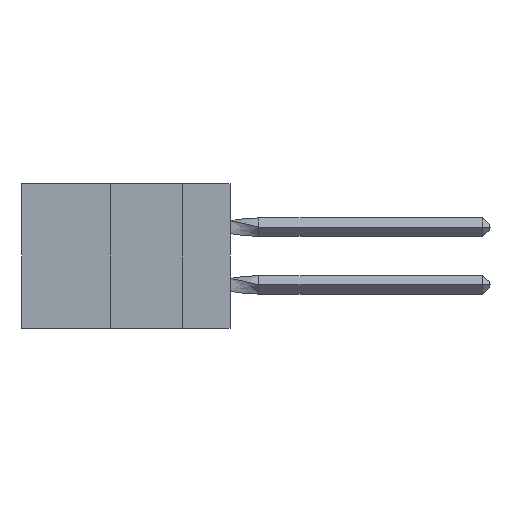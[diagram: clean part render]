
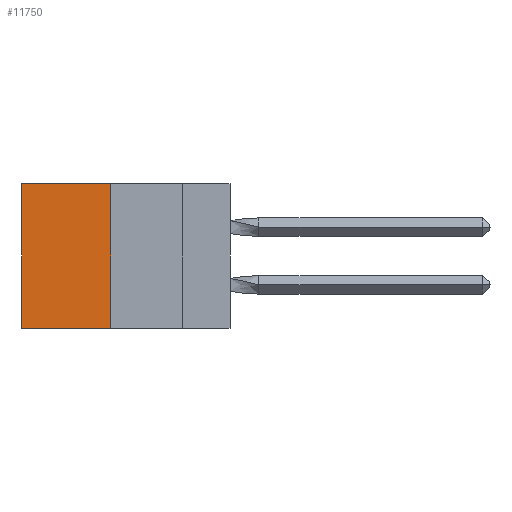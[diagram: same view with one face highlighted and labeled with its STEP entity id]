
A CAD part, left-side view. The second image highlights one B-rep face of the part: STEP entity #11750.
In plain terms, the highlighted planar face has unit normal (-1, 0, 0).
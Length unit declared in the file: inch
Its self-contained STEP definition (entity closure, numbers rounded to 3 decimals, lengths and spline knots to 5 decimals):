
#335 = DIRECTION ( 'NONE',  ( 0., 1., 0. ) ) ;
#405 = ORIENTED_EDGE ( 'NONE', *, *, #6622, .T. ) ;
#2825 = EDGE_CURVE ( 'NONE', #12807, #5251, #27028, .T. ) ;
#3251 = PLANE ( 'NONE',  #20923 ) ;
#3569 = DIRECTION ( 'NONE',  ( 0., 1., 0. ) ) ;
#4376 = CARTESIAN_POINT ( 'NONE',  ( 0.305, 0.413, -0.5 ) ) ;
#5109 = VERTEX_POINT ( 'NONE', #4376 ) ;
#5149 = CARTESIAN_POINT ( 'NONE',  ( 0.305, 0.72, 0. ) ) ;
#5251 = VERTEX_POINT ( 'NONE', #5149 ) ;
#6622 = EDGE_CURVE ( 'NONE', #5251, #14571, #18319, .T. ) ;
#6667 = VECTOR ( 'NONE', #20431, 39.37008 ) ;
#6891 = FACE_OUTER_BOUND ( 'NONE', #33500, .T. ) ;
#8095 = CARTESIAN_POINT ( 'NONE',  ( 0.305, 0.413, -0.5 ) ) ;
#10696 = EDGE_CURVE ( 'NONE', #5109, #14571, #30036, .T. ) ;
#11024 = CARTESIAN_POINT ( 'NONE',  ( 0.305, 0.413, -0.5 ) ) ;
#11435 = VECTOR ( 'NONE', #13709, 39.37008 ) ;
#11750 = ADVANCED_FACE ( 'NONE', ( #6891 ), #3251, .F. ) ;
#12391 = CARTESIAN_POINT ( 'NONE',  ( 0.305, 0.72, -0.5 ) ) ;
#12807 = VERTEX_POINT ( 'NONE', #29719 ) ;
#13709 = DIRECTION ( 'NONE',  ( 0., 0., -1. ) ) ;
#14567 = ORIENTED_EDGE ( 'NONE', *, *, #19750, .F. ) ;
#14571 = VERTEX_POINT ( 'NONE', #28990 ) ;
#17619 = LINE ( 'NONE', #11024, #11435 ) ;
#18319 = LINE ( 'NONE', #12391, #6667 ) ;
#19567 = VECTOR ( 'NONE', #335, 39.37008 ) ;
#19750 = EDGE_CURVE ( 'NONE', #12807, #5109, #17619, .T. ) ;
#20431 = DIRECTION ( 'NONE',  ( 0., 0., -1. ) ) ;
#20923 = AXIS2_PLACEMENT_3D ( 'NONE', #29618, #32327, #29840 ) ;
#22363 = CARTESIAN_POINT ( 'NONE',  ( 0.305, 0.413, 0. ) ) ;
#27028 = LINE ( 'NONE', #22363, #30759 ) ;
#27085 = ORIENTED_EDGE ( 'NONE', *, *, #2825, .T. ) ;
#28990 = CARTESIAN_POINT ( 'NONE',  ( 0.305, 0.72, -0.5 ) ) ;
#29618 = CARTESIAN_POINT ( 'NONE',  ( 0.305, 0.413, -0.5 ) ) ;
#29719 = CARTESIAN_POINT ( 'NONE',  ( 0.305, 0.413, 0. ) ) ;
#29840 = DIRECTION ( 'NONE',  ( 0., 0., -1. ) ) ;
#30036 = LINE ( 'NONE', #8095, #19567 ) ;
#30759 = VECTOR ( 'NONE', #3569, 39.37008 ) ;
#32327 = DIRECTION ( 'NONE',  ( 1., 0., 0. ) ) ;
#32688 = ORIENTED_EDGE ( 'NONE', *, *, #10696, .F. ) ;
#33500 = EDGE_LOOP ( 'NONE', ( #405, #32688, #14567, #27085 ) ) ;
